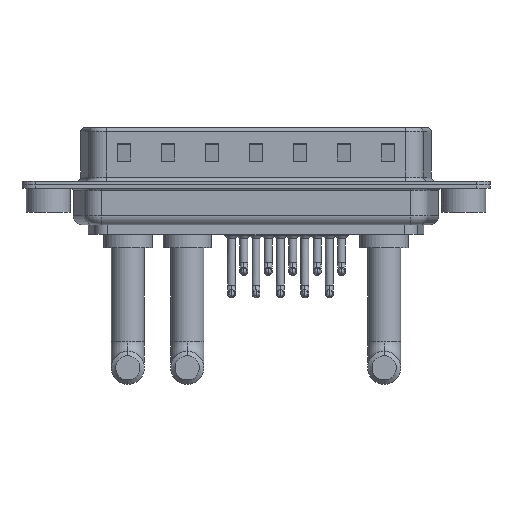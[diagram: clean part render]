
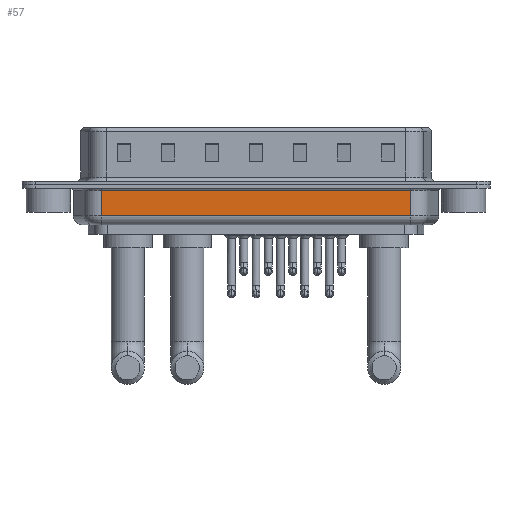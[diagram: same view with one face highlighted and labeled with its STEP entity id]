
A CAD part, front view. The second image highlights one B-rep face of the part: STEP entity #57.
In plain terms, the highlighted planar face has unit normal (0, -1, 0).
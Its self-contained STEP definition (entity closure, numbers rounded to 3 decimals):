
#57 = ADVANCED_FACE ( 'NONE', ( #13369 ), #15373, .F. ) ;
#450 = DIRECTION ( 'NONE',  ( 1., 0., 0. ) ) ;
#494 = CARTESIAN_POINT ( 'NONE',  ( 6.006, -5.35, -4.5 ) ) ;
#719 = VERTEX_POINT ( 'NONE', #23442 ) ;
#2254 = LINE ( 'NONE', #16859, #4522 ) ;
#2863 = VERTEX_POINT ( 'NONE', #20783 ) ;
#3328 = ORIENTED_EDGE ( 'NONE', *, *, #9819, .T. ) ;
#4075 = CARTESIAN_POINT ( 'NONE',  ( 41.044, -5.35, -4.5 ) ) ;
#4400 = VECTOR ( 'NONE', #13553, 1000. ) ;
#4467 = DIRECTION ( 'NONE',  ( 0., 1., 0. ) ) ;
#4522 = VECTOR ( 'NONE', #450, 1000. ) ;
#4743 = CARTESIAN_POINT ( 'NONE',  ( 6.006, -5.35, -0.65 ) ) ;
#5436 = DIRECTION ( 'NONE',  ( 0., 0., 1. ) ) ;
#5890 = LINE ( 'NONE', #4075, #16277 ) ;
#6223 = CARTESIAN_POINT ( 'NONE',  ( 6.006, -5.35, -0.65 ) ) ;
#7759 = VECTOR ( 'NONE', #16789, 1000. ) ;
#8169 = LINE ( 'NONE', #494, #7759 ) ;
#8664 = EDGE_CURVE ( 'NONE', #2863, #10917, #5890, .T. ) ;
#9819 = EDGE_CURVE ( 'NONE', #10917, #11600, #15319, .T. ) ;
#10917 = VERTEX_POINT ( 'NONE', #16321 ) ;
#11407 = ORIENTED_EDGE ( 'NONE', *, *, #8664, .T. ) ;
#11600 = VERTEX_POINT ( 'NONE', #4743 ) ;
#11652 = ORIENTED_EDGE ( 'NONE', *, *, #18316, .F. ) ;
#13369 = FACE_OUTER_BOUND ( 'NONE', #22253, .T. ) ;
#13553 = DIRECTION ( 'NONE',  ( -1., 0., 0. ) ) ;
#13926 = AXIS2_PLACEMENT_3D ( 'NONE', #22638, #4467, #15259 ) ;
#14413 = EDGE_CURVE ( 'NONE', #719, #2863, #2254, .T. ) ;
#15259 = DIRECTION ( 'NONE',  ( 0., 0., 1. ) ) ;
#15319 = LINE ( 'NONE', #6223, #4400 ) ;
#15373 = PLANE ( 'NONE',  #13926 ) ;
#16277 = VECTOR ( 'NONE', #5436, 1000. ) ;
#16321 = CARTESIAN_POINT ( 'NONE',  ( 41.044, -5.35, -0.65 ) ) ;
#16789 = DIRECTION ( 'NONE',  ( 0., 0., 1. ) ) ;
#16859 = CARTESIAN_POINT ( 'NONE',  ( 6.006, -5.35, -3.5 ) ) ;
#18316 = EDGE_CURVE ( 'NONE', #719, #11600, #8169, .T. ) ;
#20783 = CARTESIAN_POINT ( 'NONE',  ( 41.044, -5.35, -3.5 ) ) ;
#21243 = ORIENTED_EDGE ( 'NONE', *, *, #14413, .T. ) ;
#22253 = EDGE_LOOP ( 'NONE', ( #11652, #21243, #11407, #3328 ) ) ;
#22638 = CARTESIAN_POINT ( 'NONE',  ( 6.006, -5.35, -4.5 ) ) ;
#23442 = CARTESIAN_POINT ( 'NONE',  ( 6.006, -5.35, -3.5 ) ) ;
